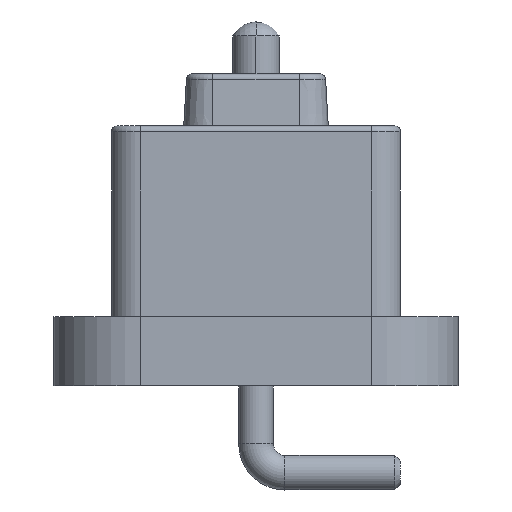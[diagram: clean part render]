
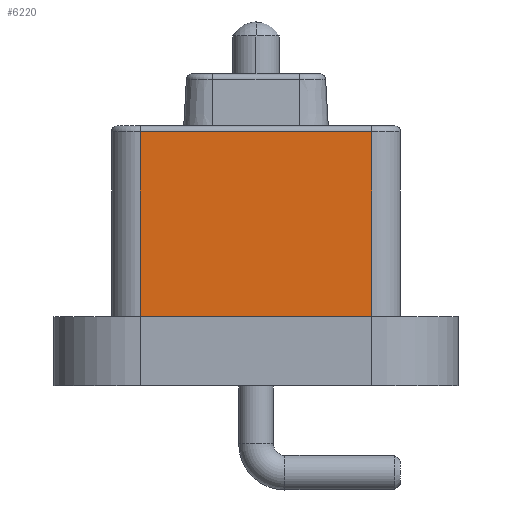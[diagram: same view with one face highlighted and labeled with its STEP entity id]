
A CAD part, left-side view. The second image highlights one B-rep face of the part: STEP entity #6220.
In plain terms, the highlighted planar face has unit normal (-1, 0, 0).
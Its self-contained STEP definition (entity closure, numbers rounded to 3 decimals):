
#484 = VERTEX_POINT ( 'NONE', #4113 ) ;
#862 = LINE ( 'NONE', #3964, #3821 ) ;
#1282 = VERTEX_POINT ( 'NONE', #8106 ) ;
#1303 = DIRECTION ( 'NONE',  ( 0., 1., 0. ) ) ;
#1335 = VECTOR ( 'NONE', #8272, 1000. ) ;
#1430 = DIRECTION ( 'NONE',  ( 1., 0., 0. ) ) ;
#1735 = EDGE_CURVE ( 'NONE', #1282, #9916, #2077, .T. ) ;
#2028 = AXIS2_PLACEMENT_3D ( 'NONE', #8387, #1430, #4525 ) ;
#2077 = LINE ( 'NONE', #5183, #1335 ) ;
#2198 = FACE_OUTER_BOUND ( 'NONE', #9749, .T. ) ;
#2683 = EDGE_CURVE ( 'NONE', #484, #1282, #862, .T. ) ;
#3264 = EDGE_CURVE ( 'NONE', #9916, #8848, #3436, .T. ) ;
#3294 = CARTESIAN_POINT ( 'NONE',  ( -9.65, -2., -0.1 ) ) ;
#3436 = LINE ( 'NONE', #6542, #7652 ) ;
#3641 = ORIENTED_EDGE ( 'NONE', *, *, #3264, .T. ) ;
#3821 = VECTOR ( 'NONE', #7063, 1000. ) ;
#3964 = CARTESIAN_POINT ( 'NONE',  ( -9.65, 2., -0.1 ) ) ;
#4113 = CARTESIAN_POINT ( 'NONE',  ( -9.65, 2., -0.1 ) ) ;
#4351 = VECTOR ( 'NONE', #1303, 1000. ) ;
#4427 = EDGE_CURVE ( 'NONE', #8848, #484, #5168, .T. ) ;
#4525 = DIRECTION ( 'NONE',  ( 0., 1., 0. ) ) ;
#4753 = ORIENTED_EDGE ( 'NONE', *, *, #1735, .T. ) ;
#5168 = LINE ( 'NONE', #8258, #4351 ) ;
#5183 = CARTESIAN_POINT ( 'NONE',  ( -9.65, 2., -3.3 ) ) ;
#5303 = PLANE ( 'NONE',  #2028 ) ;
#5600 = ORIENTED_EDGE ( 'NONE', *, *, #2683, .T. ) ;
#6220 = ADVANCED_FACE ( 'NONE', ( #2198 ), #5303, .F. ) ;
#6542 = CARTESIAN_POINT ( 'NONE',  ( -9.65, -2., -3.3 ) ) ;
#7063 = DIRECTION ( 'NONE',  ( 0., 0., -1. ) ) ;
#7247 = ORIENTED_EDGE ( 'NONE', *, *, #4427, .T. ) ;
#7652 = VECTOR ( 'NONE', #9618, 1000. ) ;
#7860 = CARTESIAN_POINT ( 'NONE',  ( -9.65, -2., -3.3 ) ) ;
#8106 = CARTESIAN_POINT ( 'NONE',  ( -9.65, 2., -3.3 ) ) ;
#8258 = CARTESIAN_POINT ( 'NONE',  ( -9.65, -2., -0.1 ) ) ;
#8272 = DIRECTION ( 'NONE',  ( 0., -1., 0. ) ) ;
#8387 = CARTESIAN_POINT ( 'NONE',  ( -9.65, 0., -1.7 ) ) ;
#8848 = VERTEX_POINT ( 'NONE', #3294 ) ;
#9618 = DIRECTION ( 'NONE',  ( 0., 0., 1. ) ) ;
#9749 = EDGE_LOOP ( 'NONE', ( #5600, #4753, #3641, #7247 ) ) ;
#9916 = VERTEX_POINT ( 'NONE', #7860 ) ;
